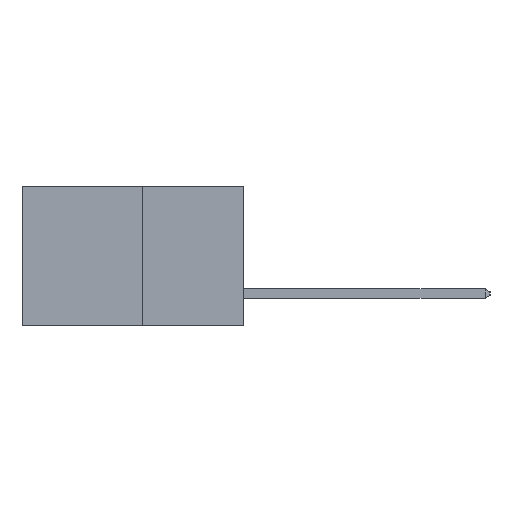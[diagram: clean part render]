
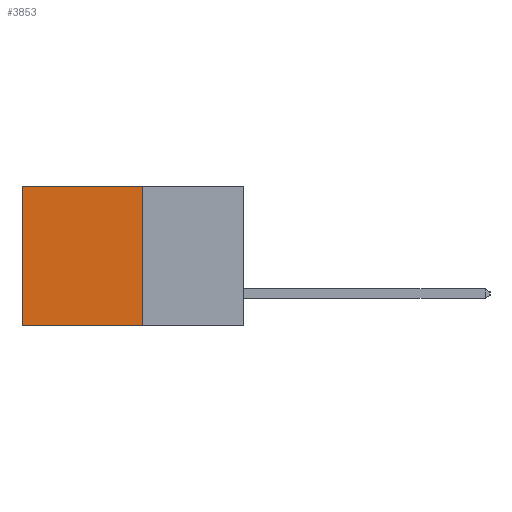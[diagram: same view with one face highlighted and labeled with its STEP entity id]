
A CAD part, left-side view. The second image highlights one B-rep face of the part: STEP entity #3853.
In plain terms, the highlighted planar face has unit normal (-1, 0, 0).
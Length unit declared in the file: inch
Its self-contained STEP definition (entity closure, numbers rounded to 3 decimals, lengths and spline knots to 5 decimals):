
#664 = EDGE_LOOP ( 'NONE', ( #9176, #8734, #7831, #1158 ) ) ;
#973 = LINE ( 'NONE', #6160, #6000 ) ;
#1158 = ORIENTED_EDGE ( 'NONE', *, *, #2458, .T. ) ;
#1247 = VERTEX_POINT ( 'NONE', #8297 ) ;
#1744 = CARTESIAN_POINT ( 'NONE',  ( 0.277, 0.59, -0.37 ) ) ;
#1888 = DIRECTION ( 'NONE',  ( 0., 0., -1. ) ) ;
#2347 = EDGE_CURVE ( 'NONE', #12016, #4089, #5203, .T. ) ;
#2458 = EDGE_CURVE ( 'NONE', #1247, #11766, #973, .T. ) ;
#2967 = VECTOR ( 'NONE', #1888, 39.37008 ) ;
#3404 = EDGE_CURVE ( 'NONE', #1247, #12016, #7967, .T. ) ;
#3706 = CARTESIAN_POINT ( 'NONE',  ( 0.277, 0.59, -0.37 ) ) ;
#3737 = LINE ( 'NONE', #3706, #5785 ) ;
#3853 = ADVANCED_FACE ( 'NONE', ( #7956 ), #6692, .F. ) ;
#3890 = DIRECTION ( 'NONE',  ( 0., 0., -1. ) ) ;
#4089 = VERTEX_POINT ( 'NONE', #1744 ) ;
#5203 = LINE ( 'NONE', #12131, #10092 ) ;
#5359 = DIRECTION ( 'NONE',  ( 0., 1., 0. ) ) ;
#5613 = EDGE_CURVE ( 'NONE', #11766, #4089, #3737, .T. ) ;
#5785 = VECTOR ( 'NONE', #3890, 39.37008 ) ;
#6000 = VECTOR ( 'NONE', #6061, 39.37008 ) ;
#6061 = DIRECTION ( 'NONE',  ( 0., 1., 0. ) ) ;
#6160 = CARTESIAN_POINT ( 'NONE',  ( 0.277, 0.27, 0. ) ) ;
#6692 = PLANE ( 'NONE',  #7175 ) ;
#6705 = CARTESIAN_POINT ( 'NONE',  ( 0.277, 0.27, -0.37 ) ) ;
#7175 = AXIS2_PLACEMENT_3D ( 'NONE', #6705, #10094, #10516 ) ;
#7831 = ORIENTED_EDGE ( 'NONE', *, *, #3404, .F. ) ;
#7956 = FACE_OUTER_BOUND ( 'NONE', #664, .T. ) ;
#7967 = LINE ( 'NONE', #8294, #2967 ) ;
#8294 = CARTESIAN_POINT ( 'NONE',  ( 0.277, 0.27, -0.37 ) ) ;
#8297 = CARTESIAN_POINT ( 'NONE',  ( 0.277, 0.27, 0. ) ) ;
#8734 = ORIENTED_EDGE ( 'NONE', *, *, #2347, .F. ) ;
#8872 = CARTESIAN_POINT ( 'NONE',  ( 0.277, 0.59, 0. ) ) ;
#9176 = ORIENTED_EDGE ( 'NONE', *, *, #5613, .T. ) ;
#10092 = VECTOR ( 'NONE', #5359, 39.37008 ) ;
#10094 = DIRECTION ( 'NONE',  ( 1., 0., 0. ) ) ;
#10516 = DIRECTION ( 'NONE',  ( 0., 0., -1. ) ) ;
#11766 = VERTEX_POINT ( 'NONE', #8872 ) ;
#12016 = VERTEX_POINT ( 'NONE', #12067 ) ;
#12067 = CARTESIAN_POINT ( 'NONE',  ( 0.277, 0.27, -0.37 ) ) ;
#12131 = CARTESIAN_POINT ( 'NONE',  ( 0.277, 0.27, -0.37 ) ) ;
